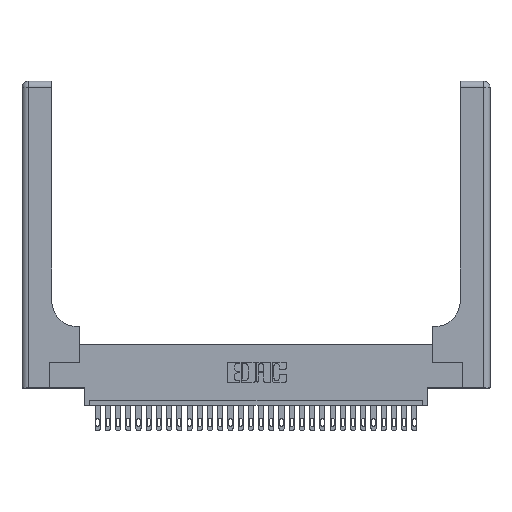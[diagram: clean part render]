
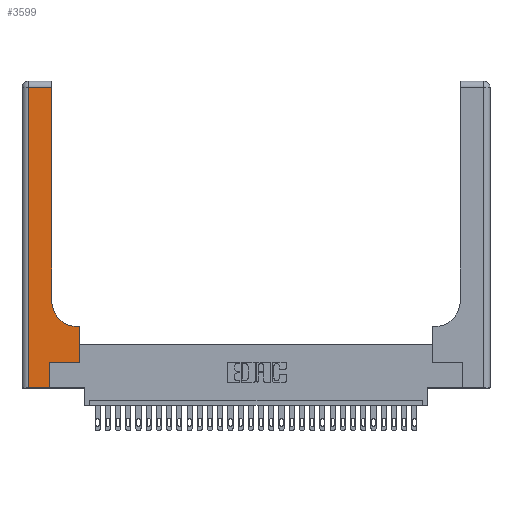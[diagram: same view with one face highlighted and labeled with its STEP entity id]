
A CAD part, top view. The second image highlights one B-rep face of the part: STEP entity #3599.
In plain terms, the highlighted planar face has unit normal (0, 0, 1).
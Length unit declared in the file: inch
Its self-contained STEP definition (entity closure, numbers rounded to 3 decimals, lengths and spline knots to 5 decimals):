
#279 = VECTOR ( 'NONE', #6816, 39.37008 ) ;
#337 = CARTESIAN_POINT ( 'NONE',  ( 0.5415, 0.85, 0.37 ) ) ;
#641 = VERTEX_POINT ( 'NONE', #3958 ) ;
#1586 = PLANE ( 'NONE',  #7009 ) ;
#3580 = LINE ( 'NONE', #30204, #279 ) ;
#3583 = DIRECTION ( 'NONE',  ( 0., 1., 0. ) ) ;
#3599 = ADVANCED_FACE ( 'NONE', ( #6228 ), #1586, .F. ) ;
#3628 = DIRECTION ( 'NONE',  ( 0., -1., 0. ) ) ;
#3870 = LINE ( 'NONE', #17723, #11681 ) ;
#3958 = CARTESIAN_POINT ( 'NONE',  ( 0.5585, 0.25, 0.37 ) ) ;
#4666 = LINE ( 'NONE', #6978, #27255 ) ;
#5063 = CARTESIAN_POINT ( 'NONE',  ( 0.5415, 0.6, 0.37 ) ) ;
#5107 = DIRECTION ( 'NONE',  ( 1., 0., 0. ) ) ;
#5220 = DIRECTION ( 'NONE',  ( 0., 0., -1. ) ) ;
#5421 = LINE ( 'NONE', #25085, #15436 ) ;
#6228 = FACE_OUTER_BOUND ( 'NONE', #14759, .T. ) ;
#6676 = VERTEX_POINT ( 'NONE', #11951 ) ;
#6816 = DIRECTION ( 'NONE',  ( 0., 1., 0. ) ) ;
#6978 = CARTESIAN_POINT ( 'NONE',  ( 0.2915, 0.6, 0.37 ) ) ;
#7009 = AXIS2_PLACEMENT_3D ( 'NONE', #25889, #5220, #28915 ) ;
#8189 = CARTESIAN_POINT ( 'NONE',  ( 0.2915, 2.94, 0.37 ) ) ;
#8622 = LINE ( 'NONE', #21715, #28257 ) ;
#8998 = ORIENTED_EDGE ( 'NONE', *, *, #21328, .T. ) ;
#9818 = ORIENTED_EDGE ( 'NONE', *, *, #21810, .T. ) ;
#10005 = DIRECTION ( 'NONE',  ( -1., 0., 0. ) ) ;
#10093 = LINE ( 'NONE', #21563, #18957 ) ;
#11681 = VECTOR ( 'NONE', #3628, 39.37008 ) ;
#11740 = EDGE_CURVE ( 'NONE', #641, #6676, #5421, .T. ) ;
#11951 = CARTESIAN_POINT ( 'NONE',  ( 0.5585, 0.6, 0.37 ) ) ;
#12137 = LINE ( 'NONE', #29809, #14351 ) ;
#12993 = ORIENTED_EDGE ( 'NONE', *, *, #11740, .T. ) ;
#13451 = EDGE_CURVE ( 'NONE', #13736, #18085, #3870, .T. ) ;
#13507 = EDGE_CURVE ( 'NONE', #25964, #641, #25334, .T. ) ;
#13736 = VERTEX_POINT ( 'NONE', #21025 ) ;
#13898 = CARTESIAN_POINT ( 'NONE',  ( 0.2915, 0.85, 0.37 ) ) ;
#14351 = VECTOR ( 'NONE', #21219, 39.37008 ) ;
#14463 = EDGE_CURVE ( 'NONE', #15276, #13736, #8622, .T. ) ;
#14759 = EDGE_LOOP ( 'NONE', ( #16800, #24476, #30302, #9818, #28509, #16563, #12993, #24120, #8998 ) ) ;
#15012 = EDGE_CURVE ( 'NONE', #23478, #25964, #10093, .T. ) ;
#15276 = VERTEX_POINT ( 'NONE', #8189 ) ;
#15436 = VECTOR ( 'NONE', #3583, 39.37008 ) ;
#16563 = ORIENTED_EDGE ( 'NONE', *, *, #13507, .T. ) ;
#16800 = ORIENTED_EDGE ( 'NONE', *, *, #24548, .T. ) ;
#16909 = DIRECTION ( 'NONE',  ( 0., 0., -1. ) ) ;
#17577 = VERTEX_POINT ( 'NONE', #13898 ) ;
#17723 = CARTESIAN_POINT ( 'NONE',  ( 0.06, 3., 0.37 ) ) ;
#18032 = CIRCLE ( 'NONE', #18237, 0.25 ) ;
#18085 = VERTEX_POINT ( 'NONE', #20855 ) ;
#18237 = AXIS2_PLACEMENT_3D ( 'NONE', #337, #16909, #5107 ) ;
#18957 = VECTOR ( 'NONE', #23519, 39.37008 ) ;
#20855 = CARTESIAN_POINT ( 'NONE',  ( 0.06, 0., 0.37 ) ) ;
#21025 = CARTESIAN_POINT ( 'NONE',  ( 0.06, 2.94, 0.37 ) ) ;
#21219 = DIRECTION ( 'NONE',  ( 1., 0., 0. ) ) ;
#21328 = EDGE_CURVE ( 'NONE', #23789, #17577, #18032, .T. ) ;
#21363 = CARTESIAN_POINT ( 'NONE',  ( 0.269, 0.25, 0.37 ) ) ;
#21563 = CARTESIAN_POINT ( 'NONE',  ( 0.269, 0., 0.37 ) ) ;
#21715 = CARTESIAN_POINT ( 'NONE',  ( 0., 2.94, 0.37 ) ) ;
#21810 = EDGE_CURVE ( 'NONE', #18085, #23478, #12137, .T. ) ;
#22034 = VECTOR ( 'NONE', #25032, 39.37008 ) ;
#23303 = DIRECTION ( 'NONE',  ( -1., 0., 0. ) ) ;
#23478 = VERTEX_POINT ( 'NONE', #27217 ) ;
#23519 = DIRECTION ( 'NONE',  ( 0., 1., 0. ) ) ;
#23789 = VERTEX_POINT ( 'NONE', #5063 ) ;
#24120 = ORIENTED_EDGE ( 'NONE', *, *, #25258, .T. ) ;
#24476 = ORIENTED_EDGE ( 'NONE', *, *, #14463, .T. ) ;
#24548 = EDGE_CURVE ( 'NONE', #17577, #15276, #3580, .T. ) ;
#25032 = DIRECTION ( 'NONE',  ( 1., 0., 0. ) ) ;
#25085 = CARTESIAN_POINT ( 'NONE',  ( 0.5585, 0.25, 0.37 ) ) ;
#25258 = EDGE_CURVE ( 'NONE', #6676, #23789, #4666, .T. ) ;
#25334 = LINE ( 'NONE', #27737, #22034 ) ;
#25889 = CARTESIAN_POINT ( 'NONE',  ( 0., 3., 0.37 ) ) ;
#25964 = VERTEX_POINT ( 'NONE', #21363 ) ;
#27217 = CARTESIAN_POINT ( 'NONE',  ( 0.269, 0., 0.37 ) ) ;
#27255 = VECTOR ( 'NONE', #23303, 39.37008 ) ;
#27737 = CARTESIAN_POINT ( 'NONE',  ( 0.269, 0.25, 0.37 ) ) ;
#28257 = VECTOR ( 'NONE', #10005, 39.37008 ) ;
#28509 = ORIENTED_EDGE ( 'NONE', *, *, #15012, .T. ) ;
#28915 = DIRECTION ( 'NONE',  ( -1., 0., 0. ) ) ;
#29809 = CARTESIAN_POINT ( 'NONE',  ( 0., 0., 0.37 ) ) ;
#30204 = CARTESIAN_POINT ( 'NONE',  ( 0.2915, 3., 0.37 ) ) ;
#30302 = ORIENTED_EDGE ( 'NONE', *, *, #13451, .T. ) ;
